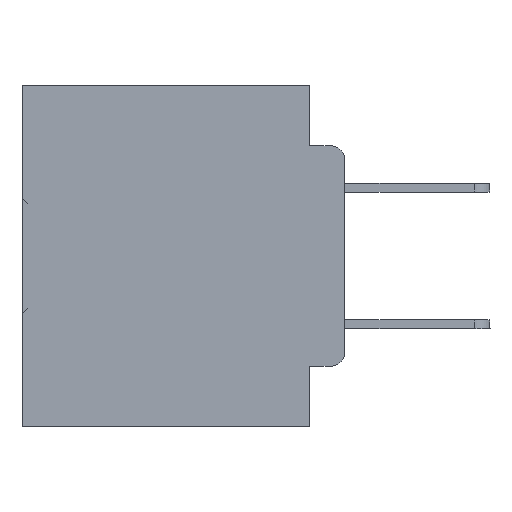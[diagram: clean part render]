
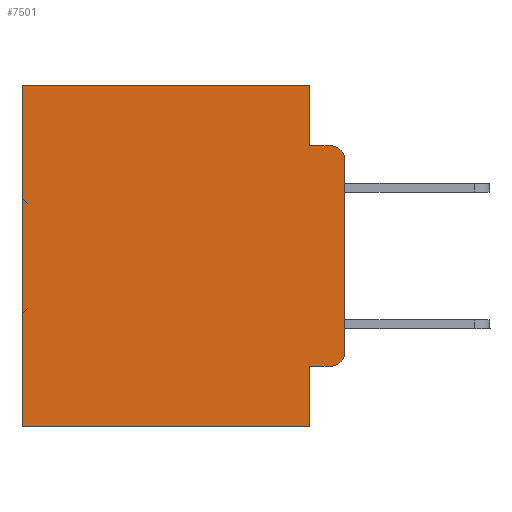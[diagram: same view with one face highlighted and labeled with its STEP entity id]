
A CAD part, left-side view. The second image highlights one B-rep face of the part: STEP entity #7501.
In plain terms, the highlighted planar face has unit normal (-1, 0, 0).
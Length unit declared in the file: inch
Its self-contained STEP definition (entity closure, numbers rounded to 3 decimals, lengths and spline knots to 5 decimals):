
#215 = VERTEX_POINT ( 'NONE', #27351 ) ;
#470 = LINE ( 'NONE', #31800, #14907 ) ;
#964 = VERTEX_POINT ( 'NONE', #11642 ) ;
#1131 = CARTESIAN_POINT ( 'NONE',  ( 0.298, 0.473, -0.5 ) ) ;
#1821 = EDGE_CURVE ( 'NONE', #964, #27178, #35948, .T. ) ;
#1848 = CARTESIAN_POINT ( 'NONE',  ( 0.298, 0.02, -0.0885 ) ) ;
#1868 = CARTESIAN_POINT ( 'NONE',  ( 0.298, 0.051, -0.4115 ) ) ;
#1924 = DIRECTION ( 'NONE',  ( 0., 0., -1. ) ) ;
#2959 = LINE ( 'NONE', #25474, #10689 ) ;
#3251 = VECTOR ( 'NONE', #24731, 39.37008 ) ;
#3363 = EDGE_CURVE ( 'NONE', #14856, #964, #470, .T. ) ;
#3839 = DIRECTION ( 'NONE',  ( 1., 0., 0. ) ) ;
#4733 = DIRECTION ( 'NONE',  ( -1., 0., 0. ) ) ;
#4823 = CARTESIAN_POINT ( 'NONE',  ( 0.298, 0.051, -0.0885 ) ) ;
#4949 = VECTOR ( 'NONE', #12875, 39.37008 ) ;
#5234 = DIRECTION ( 'NONE',  ( 0., 0., -1. ) ) ;
#5681 = VERTEX_POINT ( 'NONE', #31126 ) ;
#5858 = ORIENTED_EDGE ( 'NONE', *, *, #1821, .T. ) ;
#6053 = CARTESIAN_POINT ( 'NONE',  ( 0.298, 0.051, -0.4115 ) ) ;
#7058 = ORIENTED_EDGE ( 'NONE', *, *, #23525, .F. ) ;
#7239 = VERTEX_POINT ( 'NONE', #4823 ) ;
#7417 = VECTOR ( 'NONE', #14809, 39.37008 ) ;
#7501 = ADVANCED_FACE ( 'NONE', ( #21283 ), #20917, .F. ) ;
#7617 = DIRECTION ( 'NONE',  ( 0., 0., -1. ) ) ;
#7731 = EDGE_CURVE ( 'NONE', #36792, #20055, #13399, .T. ) ;
#8771 = AXIS2_PLACEMENT_3D ( 'NONE', #35694, #4733, #1924 ) ;
#8898 = DIRECTION ( 'NONE',  ( 0., 1., 0. ) ) ;
#9468 = VECTOR ( 'NONE', #7617, 39.37008 ) ;
#10221 = DIRECTION ( 'NONE',  ( 0., 0., -1. ) ) ;
#10689 = VECTOR ( 'NONE', #5234, 39.37008 ) ;
#10805 = CARTESIAN_POINT ( 'NONE',  ( 0.298, 0.473, 0. ) ) ;
#11577 = CARTESIAN_POINT ( 'NONE',  ( 0.298, 0.051, -0.5 ) ) ;
#11633 = ORIENTED_EDGE ( 'NONE', *, *, #28661, .T. ) ;
#11642 = CARTESIAN_POINT ( 'NONE',  ( 0.298, 0.473, 0. ) ) ;
#12433 = EDGE_CURVE ( 'NONE', #14856, #7239, #2959, .T. ) ;
#12875 = DIRECTION ( 'NONE',  ( 0., 1., 0. ) ) ;
#13399 = LINE ( 'NONE', #36307, #27844 ) ;
#13400 = CIRCLE ( 'NONE', #19969, 0.02 ) ;
#13576 = CIRCLE ( 'NONE', #8771, 0.02 ) ;
#13800 = ORIENTED_EDGE ( 'NONE', *, *, #35878, .T. ) ;
#14650 = VERTEX_POINT ( 'NONE', #28858 ) ;
#14809 = DIRECTION ( 'NONE',  ( 0., -1., 0. ) ) ;
#14856 = VERTEX_POINT ( 'NONE', #25213 ) ;
#14907 = VECTOR ( 'NONE', #8898, 39.37008 ) ;
#14940 = ORIENTED_EDGE ( 'NONE', *, *, #7731, .F. ) ;
#15502 = DIRECTION ( 'NONE',  ( -1., 0., 0. ) ) ;
#18488 = LINE ( 'NONE', #32595, #4949 ) ;
#18630 = VERTEX_POINT ( 'NONE', #1848 ) ;
#19230 = DIRECTION ( 'NONE',  ( 0., 0., -1. ) ) ;
#19587 = LINE ( 'NONE', #31063, #29547 ) ;
#19969 = AXIS2_PLACEMENT_3D ( 'NONE', #26585, #15502, #26956 ) ;
#20034 = AXIS2_PLACEMENT_3D ( 'NONE', #20534, #3839, #34991 ) ;
#20055 = VERTEX_POINT ( 'NONE', #11577 ) ;
#20534 = CARTESIAN_POINT ( 'NONE',  ( 0.298, 0., 0. ) ) ;
#20917 = PLANE ( 'NONE',  #20034 ) ;
#21283 = FACE_OUTER_BOUND ( 'NONE', #31263, .T. ) ;
#23525 = EDGE_CURVE ( 'NONE', #5681, #215, #19587, .T. ) ;
#24522 = ORIENTED_EDGE ( 'NONE', *, *, #26074, .T. ) ;
#24594 = EDGE_CURVE ( 'NONE', #20055, #27178, #18488, .T. ) ;
#24731 = DIRECTION ( 'NONE',  ( 0., -1., 0. ) ) ;
#25213 = CARTESIAN_POINT ( 'NONE',  ( 0.298, 0.051, 0. ) ) ;
#25474 = CARTESIAN_POINT ( 'NONE',  ( 0.298, 0.051, 0. ) ) ;
#25833 = EDGE_CURVE ( 'NONE', #7239, #18630, #25879, .T. ) ;
#25879 = LINE ( 'NONE', #34523, #7417 ) ;
#26074 = EDGE_CURVE ( 'NONE', #36792, #14650, #36019, .T. ) ;
#26585 = CARTESIAN_POINT ( 'NONE',  ( 0.298, 0.02, -0.3915 ) ) ;
#26956 = DIRECTION ( 'NONE',  ( 0., 0., -1. ) ) ;
#27104 = ORIENTED_EDGE ( 'NONE', *, *, #12433, .F. ) ;
#27178 = VERTEX_POINT ( 'NONE', #1131 ) ;
#27351 = CARTESIAN_POINT ( 'NONE',  ( 0.298, 0., -0.3915 ) ) ;
#27844 = VECTOR ( 'NONE', #10221, 39.37008 ) ;
#28661 = EDGE_CURVE ( 'NONE', #5681, #18630, #13576, .T. ) ;
#28831 = ORIENTED_EDGE ( 'NONE', *, *, #24594, .F. ) ;
#28858 = CARTESIAN_POINT ( 'NONE',  ( 0.298, 0.02, -0.4115 ) ) ;
#29547 = VECTOR ( 'NONE', #19230, 39.37008 ) ;
#30584 = ORIENTED_EDGE ( 'NONE', *, *, #25833, .F. ) ;
#30802 = ORIENTED_EDGE ( 'NONE', *, *, #3363, .T. ) ;
#31063 = CARTESIAN_POINT ( 'NONE',  ( 0.298, 0., 0. ) ) ;
#31126 = CARTESIAN_POINT ( 'NONE',  ( 0.298, 0., -0.1085 ) ) ;
#31263 = EDGE_LOOP ( 'NONE', ( #7058, #11633, #30584, #27104, #30802, #5858, #28831, #14940, #24522, #13800 ) ) ;
#31800 = CARTESIAN_POINT ( 'NONE',  ( 0.298, 0., 0. ) ) ;
#32595 = CARTESIAN_POINT ( 'NONE',  ( 0.298, 0., -0.5 ) ) ;
#34523 = CARTESIAN_POINT ( 'NONE',  ( 0.298, 0.051, -0.0885 ) ) ;
#34991 = DIRECTION ( 'NONE',  ( 0., 0., -1. ) ) ;
#35694 = CARTESIAN_POINT ( 'NONE',  ( 0.298, 0.02, -0.1085 ) ) ;
#35878 = EDGE_CURVE ( 'NONE', #14650, #215, #13400, .T. ) ;
#35948 = LINE ( 'NONE', #10805, #9468 ) ;
#36019 = LINE ( 'NONE', #1868, #3251 ) ;
#36307 = CARTESIAN_POINT ( 'NONE',  ( 0.298, 0.051, 0. ) ) ;
#36792 = VERTEX_POINT ( 'NONE', #6053 ) ;
